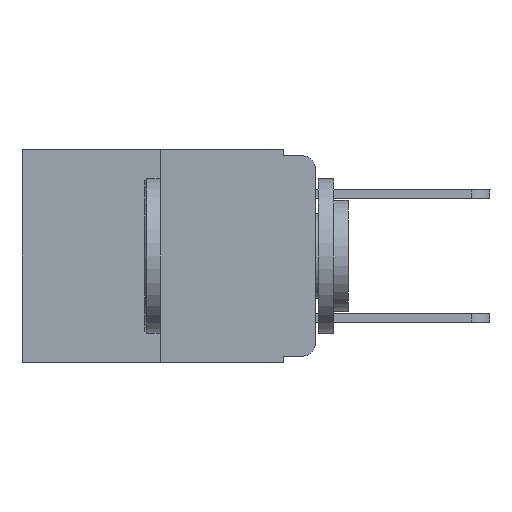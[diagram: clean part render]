
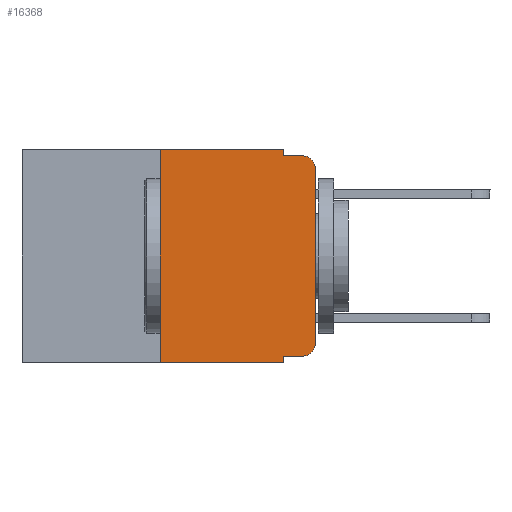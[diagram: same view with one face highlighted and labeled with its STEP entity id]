
A CAD part, left-side view. The second image highlights one B-rep face of the part: STEP entity #16368.
In plain terms, the highlighted planar face has unit normal (-1, 0, 0).
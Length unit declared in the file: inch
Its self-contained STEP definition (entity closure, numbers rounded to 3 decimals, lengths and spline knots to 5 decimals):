
#292 = VECTOR ( 'NONE', #22222, 39.37008 ) ;
#573 = VECTOR ( 'NONE', #22177, 39.37008 ) ;
#1507 = VERTEX_POINT ( 'NONE', #10015 ) ;
#1584 = EDGE_CURVE ( 'NONE', #20631, #13913, #8461, .T. ) ;
#1917 = VERTEX_POINT ( 'NONE', #17563 ) ;
#2261 = DIRECTION ( 'NONE',  ( 0., -1., 0. ) ) ;
#2267 = LINE ( 'NONE', #4205, #11925 ) ;
#2451 = VECTOR ( 'NONE', #6526, 39.37008 ) ;
#2793 = DIRECTION ( 'NONE',  ( 0., 0., -1. ) ) ;
#3329 = EDGE_CURVE ( 'NONE', #1507, #3457, #2267, .T. ) ;
#3457 = VERTEX_POINT ( 'NONE', #22430 ) ;
#3586 = FACE_OUTER_BOUND ( 'NONE', #21516, .T. ) ;
#4205 = CARTESIAN_POINT ( 'NONE',  ( 0., 0.051, 0. ) ) ;
#4251 = LINE ( 'NONE', #5821, #15795 ) ;
#4424 = CARTESIAN_POINT ( 'NONE',  ( 0., 0.051, 0. ) ) ;
#4830 = ORIENTED_EDGE ( 'NONE', *, *, #12105, .F. ) ;
#5317 = VECTOR ( 'NONE', #2793, 39.37008 ) ;
#5334 = CARTESIAN_POINT ( 'NONE',  ( 0., 0.25, 0. ) ) ;
#5426 = VERTEX_POINT ( 'NONE', #5334 ) ;
#5572 = CARTESIAN_POINT ( 'NONE',  ( 0., 0.02, -0.01 ) ) ;
#5636 = ORIENTED_EDGE ( 'NONE', *, *, #1584, .T. ) ;
#5821 = CARTESIAN_POINT ( 'NONE',  ( 0., 0.473, -0.343 ) ) ;
#5891 = DIRECTION ( 'NONE',  ( 0., 0., -1. ) ) ;
#6026 = VERTEX_POINT ( 'NONE', #16734 ) ;
#6191 = EDGE_CURVE ( 'NONE', #1917, #22500, #10166, .T. ) ;
#6526 = DIRECTION ( 'NONE',  ( 0., 0., 1. ) ) ;
#6558 = CARTESIAN_POINT ( 'NONE',  ( 0., 0.051, -0.01 ) ) ;
#6642 = EDGE_CURVE ( 'NONE', #6026, #20631, #24880, .T. ) ;
#7424 = DIRECTION ( 'NONE',  ( -1., 0., 0. ) ) ;
#8461 = LINE ( 'NONE', #16044, #2451 ) ;
#8569 = LINE ( 'NONE', #10370, #16306 ) ;
#9944 = ORIENTED_EDGE ( 'NONE', *, *, #22482, .T. ) ;
#10015 = CARTESIAN_POINT ( 'NONE',  ( 0., 0.051, -0.333 ) ) ;
#10086 = EDGE_CURVE ( 'NONE', #23812, #3457, #4251, .T. ) ;
#10166 = LINE ( 'NONE', #6558, #292 ) ;
#10370 = CARTESIAN_POINT ( 'NONE',  ( 0., 0.051, -0.333 ) ) ;
#10496 = CIRCLE ( 'NONE', #23190, 0.02 ) ;
#10992 = CARTESIAN_POINT ( 'NONE',  ( 0., 0., -0.03 ) ) ;
#11419 = CARTESIAN_POINT ( 'NONE',  ( 0., 0.473, 0. ) ) ;
#11925 = VECTOR ( 'NONE', #5891, 39.37008 ) ;
#12105 = EDGE_CURVE ( 'NONE', #5426, #23692, #20497, .T. ) ;
#12198 = ORIENTED_EDGE ( 'NONE', *, *, #10086, .T. ) ;
#12429 = CARTESIAN_POINT ( 'NONE',  ( 0., 0.02, -0.313 ) ) ;
#13249 = AXIS2_PLACEMENT_3D ( 'NONE', #11419, #17071, #17583 ) ;
#13424 = EDGE_CURVE ( 'NONE', #13913, #22500, #10496, .T. ) ;
#13450 = EDGE_CURVE ( 'NONE', #23812, #5426, #23080, .T. ) ;
#13913 = VERTEX_POINT ( 'NONE', #10992 ) ;
#14487 = CARTESIAN_POINT ( 'NONE',  ( 0., 0.473, 0. ) ) ;
#15319 = ORIENTED_EDGE ( 'NONE', *, *, #6642, .T. ) ;
#15795 = VECTOR ( 'NONE', #23770, 39.37008 ) ;
#16044 = CARTESIAN_POINT ( 'NONE',  ( 0., 0., 0. ) ) ;
#16306 = VECTOR ( 'NONE', #2261, 39.37008 ) ;
#16366 = CARTESIAN_POINT ( 'NONE',  ( 0., 0.25, -0.343 ) ) ;
#16368 = ADVANCED_FACE ( 'NONE', ( #3586 ), #19121, .F. ) ;
#16419 = DIRECTION ( 'NONE',  ( 0., 0., -1. ) ) ;
#16734 = CARTESIAN_POINT ( 'NONE',  ( 0., 0.02, -0.333 ) ) ;
#17071 = DIRECTION ( 'NONE',  ( 1., 0., 0. ) ) ;
#17435 = DIRECTION ( 'NONE',  ( 0., 0., 1. ) ) ;
#17563 = CARTESIAN_POINT ( 'NONE',  ( 0., 0.051, -0.01 ) ) ;
#17583 = DIRECTION ( 'NONE',  ( 0., 0., -1. ) ) ;
#17616 = ORIENTED_EDGE ( 'NONE', *, *, #13450, .F. ) ;
#18025 = EDGE_CURVE ( 'NONE', #23692, #1917, #24376, .T. ) ;
#18279 = VECTOR ( 'NONE', #17435, 39.37008 ) ;
#19121 = PLANE ( 'NONE',  #13249 ) ;
#19755 = DIRECTION ( 'NONE',  ( -1., 0., 0. ) ) ;
#19920 = ORIENTED_EDGE ( 'NONE', *, *, #3329, .F. ) ;
#20497 = LINE ( 'NONE', #14487, #573 ) ;
#20631 = VERTEX_POINT ( 'NONE', #22670 ) ;
#21516 = EDGE_LOOP ( 'NONE', ( #5636, #24339, #23092, #24958, #4830, #17616, #12198, #19920, #9944, #15319 ) ) ;
#21577 = AXIS2_PLACEMENT_3D ( 'NONE', #12429, #19755, #16419 ) ;
#22177 = DIRECTION ( 'NONE',  ( 0., -1., 0. ) ) ;
#22222 = DIRECTION ( 'NONE',  ( 0., -1., 0. ) ) ;
#22313 = CARTESIAN_POINT ( 'NONE',  ( 0., 0.051, 0. ) ) ;
#22430 = CARTESIAN_POINT ( 'NONE',  ( 0., 0.051, -0.343 ) ) ;
#22482 = EDGE_CURVE ( 'NONE', #1507, #6026, #8569, .T. ) ;
#22500 = VERTEX_POINT ( 'NONE', #5572 ) ;
#22670 = CARTESIAN_POINT ( 'NONE',  ( 0., 0., -0.313 ) ) ;
#22823 = CARTESIAN_POINT ( 'NONE',  ( 0., 0.02, -0.03 ) ) ;
#23080 = LINE ( 'NONE', #23332, #18279 ) ;
#23092 = ORIENTED_EDGE ( 'NONE', *, *, #6191, .F. ) ;
#23190 = AXIS2_PLACEMENT_3D ( 'NONE', #22823, #7424, #25006 ) ;
#23332 = CARTESIAN_POINT ( 'NONE',  ( 0., 0.25, 0. ) ) ;
#23692 = VERTEX_POINT ( 'NONE', #4424 ) ;
#23770 = DIRECTION ( 'NONE',  ( 0., -1., 0. ) ) ;
#23812 = VERTEX_POINT ( 'NONE', #16366 ) ;
#24339 = ORIENTED_EDGE ( 'NONE', *, *, #13424, .T. ) ;
#24376 = LINE ( 'NONE', #22313, #5317 ) ;
#24880 = CIRCLE ( 'NONE', #21577, 0.02 ) ;
#24958 = ORIENTED_EDGE ( 'NONE', *, *, #18025, .F. ) ;
#25006 = DIRECTION ( 'NONE',  ( 0., 0., -1. ) ) ;
